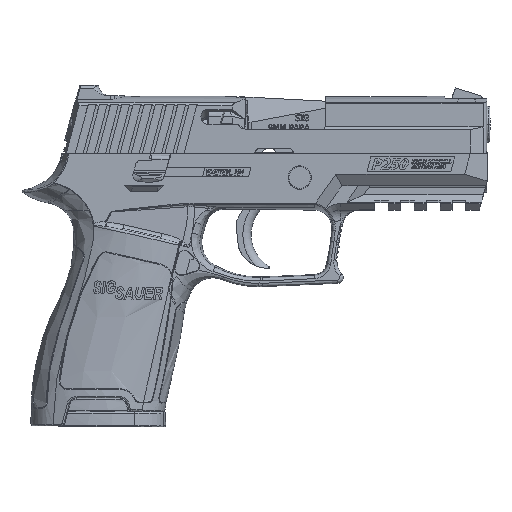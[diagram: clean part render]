
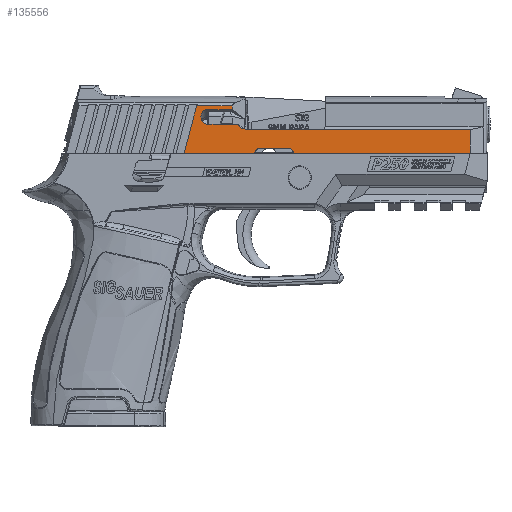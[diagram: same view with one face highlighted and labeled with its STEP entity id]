
A CAD part, top view. The second image highlights one B-rep face of the part: STEP entity #135556.
In plain terms, the highlighted planar face has unit normal (0, 0, 1).
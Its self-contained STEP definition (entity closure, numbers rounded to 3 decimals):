
#2922 = EDGE_CURVE ( 'NONE', #13814, #132730, #89528, .T. ) ;
#5060 = CARTESIAN_POINT ( 'NONE',  ( 76.306, -5.512, 13.392 ) ) ;
#7106 = CARTESIAN_POINT ( 'NONE',  ( -25.864, 5.823, 13.392 ) ) ;
#8354 = LINE ( 'NONE', #92009, #197966 ) ;
#10032 = VECTOR ( 'NONE', #90291, 1000. ) ;
#10388 = DIRECTION ( 'NONE',  ( -1., 0., 0. ) ) ;
#10726 = CIRCLE ( 'NONE', #40837, 1.892 ) ;
#12223 = VECTOR ( 'NONE', #10388, 1000. ) ;
#13460 = DIRECTION ( 'NONE',  ( 1., 0., 0. ) ) ;
#13528 = DIRECTION ( 'NONE',  ( 0., 0., -1. ) ) ;
#13814 = VERTEX_POINT ( 'NONE', #211452 ) ;
#14799 = CARTESIAN_POINT ( 'NONE',  ( 76.306, -1.88, 13.392 ) ) ;
#18044 = LINE ( 'NONE', #211913, #12223 ) ;
#18576 = VECTOR ( 'NONE', #13460, 1000. ) ;
#20163 = CARTESIAN_POINT ( 'NONE',  ( -16.059, 7.282, 13.392 ) ) ;
#24333 = LINE ( 'NONE', #105023, #18576 ) ;
#29088 = VECTOR ( 'NONE', #121950, 1000. ) ;
#29481 = VERTEX_POINT ( 'NONE', #107072 ) ;
#31237 = DIRECTION ( 'NONE',  ( 0., 1., 0. ) ) ;
#31293 = DIRECTION ( 'NONE',  ( 0., 0., -1. ) ) ;
#32846 = VERTEX_POINT ( 'NONE', #14799 ) ;
#38443 = CARTESIAN_POINT ( 'NONE',  ( -11.049, -1.88, 13.392 ) ) ;
#40493 = EDGE_CURVE ( 'NONE', #134322, #143446, #10726, .T. ) ;
#40837 = AXIS2_PLACEMENT_3D ( 'NONE', #123600, #13528, #142074 ) ;
#45986 = LINE ( 'NONE', #68827, #132365 ) ;
#46815 = AXIS2_PLACEMENT_3D ( 'NONE', #141336, #31293, #159759 ) ;
#49719 = CARTESIAN_POINT ( 'NONE',  ( -11.049, 1.499, 13.392 ) ) ;
#50342 = EDGE_CURVE ( 'NONE', #98184, #13814, #45986, .T. ) ;
#51182 = CARTESIAN_POINT ( 'NONE',  ( -33.313, -5.74, 13.392 ) ) ;
#51683 = CARTESIAN_POINT ( 'NONE',  ( 18.479, -1.88, 13.392 ) ) ;
#51698 = ORIENTED_EDGE ( 'NONE', *, *, #138721, .T. ) ;
#51825 = EDGE_CURVE ( 'NONE', #29481, #180648, #100212, .T. ) ;
#55468 = ORIENTED_EDGE ( 'NONE', *, *, #212171, .T. ) ;
#60237 = ORIENTED_EDGE ( 'NONE', *, *, #66510, .T. ) ;
#60846 = EDGE_CURVE ( 'NONE', #177034, #98184, #181710, .T. ) ;
#61339 = EDGE_CURVE ( 'NONE', #132730, #151941, #153221, .T. ) ;
#61347 = DIRECTION ( 'NONE',  ( 1., 0., 0. ) ) ;
#64230 = CARTESIAN_POINT ( 'NONE',  ( -30.436, 0.241, 13.392 ) ) ;
#66371 = LINE ( 'NONE', #51182, #29088 ) ;
#66510 = EDGE_CURVE ( 'NONE', #108976, #29481, #200389, .T. ) ;
#68212 = DIRECTION ( 'NONE',  ( -0.574, -0.819, 0. ) ) ;
#68827 = CARTESIAN_POINT ( 'NONE',  ( -11.049, 5.512, 13.392 ) ) ;
#71782 = CARTESIAN_POINT ( 'NONE',  ( 0., 5.823, 13.392 ) ) ;
#73894 = VERTEX_POINT ( 'NONE', #20163 ) ;
#76267 = ORIENTED_EDGE ( 'NONE', *, *, #149920, .T. ) ;
#78929 = CARTESIAN_POINT ( 'NONE',  ( -5.524, -1.88, 13.392 ) ) ;
#79886 = ORIENTED_EDGE ( 'NONE', *, *, #177039, .T. ) ;
#82765 = CARTESIAN_POINT ( 'NONE',  ( -30.436, 5.823, 13.392 ) ) ;
#84034 = VECTOR ( 'NONE', #188940, 1000. ) ;
#86768 = VERTEX_POINT ( 'NONE', #7106 ) ;
#87944 = EDGE_CURVE ( 'NONE', #211106, #134322, #24333, .T. ) ;
#89528 = CIRCLE ( 'NONE', #101850, 3.175 ) ;
#90291 = DIRECTION ( 'NONE',  ( 1., 0., 0. ) ) ;
#92009 = CARTESIAN_POINT ( 'NONE',  ( -10.287, 7.282, 13.392 ) ) ;
#92704 = EDGE_CURVE ( 'NONE', #143446, #108976, #215526, .T. ) ;
#93083 = CARTESIAN_POINT ( 'NONE',  ( -25.864, 0.241, 13.392 ) ) ;
#94252 = EDGE_CURVE ( 'NONE', #129541, #73894, #134827, .T. ) ;
#98107 = CARTESIAN_POINT ( 'NONE',  ( -29.824, 7.282, 13.392 ) ) ;
#98184 = VERTEX_POINT ( 'NONE', #38443 ) ;
#100212 = LINE ( 'NONE', #238475, #105996 ) ;
#101850 = AXIS2_PLACEMENT_3D ( 'NONE', #49719, #178216, #68212 ) ;
#104007 = EDGE_CURVE ( 'NONE', #32846, #177034, #18044, .T. ) ;
#105023 = CARTESIAN_POINT ( 'NONE',  ( 82.626, -11.024, 13.392 ) ) ;
#105996 = VECTOR ( 'NONE', #165419, 1000. ) ;
#106846 = VECTOR ( 'NONE', #172543, 1000. ) ;
#107072 = CARTESIAN_POINT ( 'NONE',  ( 7.696, -11.024, 13.392 ) ) ;
#108976 = VERTEX_POINT ( 'NONE', #150708 ) ;
#115071 = DIRECTION ( 'NONE',  ( 0., 1., 0. ) ) ;
#121950 = DIRECTION ( 'NONE',  ( -0.259, -0.966, 0. ) ) ;
#123600 = CARTESIAN_POINT ( 'NONE',  ( -5.347, -11.024, 13.392 ) ) ;
#126146 = ORIENTED_EDGE ( 'NONE', *, *, #94252, .T. ) ;
#126937 = EDGE_CURVE ( 'NONE', #180648, #32846, #166859, .T. ) ;
#127649 = DIRECTION ( 'NONE',  ( 1., 0., 0. ) ) ;
#129541 = VERTEX_POINT ( 'NONE', #170852 ) ;
#132365 = VECTOR ( 'NONE', #161971, 1000. ) ;
#132730 = VERTEX_POINT ( 'NONE', #227591 ) ;
#134322 = VERTEX_POINT ( 'NONE', #145056 ) ;
#134827 = LINE ( 'NONE', #141280, #183573 ) ;
#135556 = ADVANCED_FACE ( 'NONE', ( #208088 ), #219091, .T. ) ;
#138721 = EDGE_CURVE ( 'NONE', #147623, #211106, #66371, .T. ) ;
#139306 = CARTESIAN_POINT ( 'NONE',  ( -34.729, -11.024, 13.392 ) ) ;
#141280 = CARTESIAN_POINT ( 'NONE',  ( -16.059, 4.602, 13.392 ) ) ;
#141336 = CARTESIAN_POINT ( 'NONE',  ( 5.804, -11.024, 13.392 ) ) ;
#142074 = DIRECTION ( 'NONE',  ( 0., 1., 0. ) ) ;
#142079 = EDGE_LOOP ( 'NONE', ( #76267, #51698, #184163, #158860, #164573, #60237, #157191, #203242, #181123, #195046, #209443, #165718, #181007, #55468, #79886, #126146 ) ) ;
#143446 = VERTEX_POINT ( 'NONE', #213743 ) ;
#145056 = CARTESIAN_POINT ( 'NONE',  ( -7.239, -11.024, 13.392 ) ) ;
#147623 = VERTEX_POINT ( 'NONE', #98107 ) ;
#149920 = EDGE_CURVE ( 'NONE', #73894, #147623, #8354, .T. ) ;
#150708 = CARTESIAN_POINT ( 'NONE',  ( 5.804, -9.131, 13.392 ) ) ;
#151941 = VERTEX_POINT ( 'NONE', #93083 ) ;
#153221 = LINE ( 'NONE', #190978, #106846 ) ;
#156608 = LINE ( 'NONE', #71782, #10032 ) ;
#157191 = ORIENTED_EDGE ( 'NONE', *, *, #51825, .T. ) ;
#158860 = ORIENTED_EDGE ( 'NONE', *, *, #40493, .T. ) ;
#159759 = DIRECTION ( 'NONE',  ( 1., 0., 0. ) ) ;
#160980 = VECTOR ( 'NONE', #61347, 1000. ) ;
#161971 = DIRECTION ( 'NONE',  ( 0., 1., 0. ) ) ;
#163719 = CARTESIAN_POINT ( 'NONE',  ( 0., 0., 13.392 ) ) ;
#164573 = ORIENTED_EDGE ( 'NONE', *, *, #92704, .T. ) ;
#165419 = DIRECTION ( 'NONE',  ( 1., 0., 0. ) ) ;
#165718 = ORIENTED_EDGE ( 'NONE', *, *, #2922, .T. ) ;
#165897 = DIRECTION ( 'NONE',  ( -1., 0., 0. ) ) ;
#166859 = LINE ( 'NONE', #5060, #172572 ) ;
#170852 = CARTESIAN_POINT ( 'NONE',  ( -16.059, 5.823, 13.392 ) ) ;
#172543 = DIRECTION ( 'NONE',  ( -1., 0., 0. ) ) ;
#172572 = VECTOR ( 'NONE', #115071, 1000. ) ;
#174250 = CARTESIAN_POINT ( 'NONE',  ( -25.864, 0.241, 13.392 ) ) ;
#177034 = VERTEX_POINT ( 'NONE', #51683 ) ;
#177039 = EDGE_CURVE ( 'NONE', #86768, #129541, #156608, .T. ) ;
#178216 = DIRECTION ( 'NONE',  ( 0., 0., -1. ) ) ;
#180648 = VERTEX_POINT ( 'NONE', #224640 ) ;
#181007 = ORIENTED_EDGE ( 'NONE', *, *, #61339, .T. ) ;
#181123 = ORIENTED_EDGE ( 'NONE', *, *, #104007, .T. ) ;
#181710 = LINE ( 'NONE', #78929, #84034 ) ;
#183573 = VECTOR ( 'NONE', #31237, 1000. ) ;
#184163 = ORIENTED_EDGE ( 'NONE', *, *, #87944, .T. ) ;
#188940 = DIRECTION ( 'NONE',  ( -1., 0., 0. ) ) ;
#190978 = CARTESIAN_POINT ( 'NONE',  ( 0., 0.241, 13.392 ) ) ;
#195046 = ORIENTED_EDGE ( 'NONE', *, *, #60846, .T. ) ;
#197966 = VECTOR ( 'NONE', #165897, 1000. ) ;
#200389 = CIRCLE ( 'NONE', #46815, 1.892 ) ;
#203242 = ORIENTED_EDGE ( 'NONE', *, *, #126937, .T. ) ;
#206339 =( BOUNDED_CURVE ( )  B_SPLINE_CURVE ( 3, ( #174250, #64230, #82765, #211164 ),
 .UNSPECIFIED., .F., .T. ) 
 B_SPLINE_CURVE_WITH_KNOTS ( ( 4, 4 ),
 ( 3.142, 6.283 ),
 .UNSPECIFIED. ) 
 CURVE ( )  GEOMETRIC_REPRESENTATION_ITEM ( )  RATIONAL_B_SPLINE_CURVE ( ( 1., 0.333, 0.333, 1. ) ) 
 REPRESENTATION_ITEM ( '' )  );
#208088 = FACE_OUTER_BOUND ( 'NONE', #142079, .T. ) ;
#209113 = CARTESIAN_POINT ( 'NONE',  ( -2.673, -9.131, 13.392 ) ) ;
#209443 = ORIENTED_EDGE ( 'NONE', *, *, #50342, .T. ) ;
#211106 = VERTEX_POINT ( 'NONE', #139306 ) ;
#211164 = CARTESIAN_POINT ( 'NONE',  ( -25.864, 5.823, 13.392 ) ) ;
#211452 = CARTESIAN_POINT ( 'NONE',  ( -11.049, -1.676, 13.392 ) ) ;
#211913 = CARTESIAN_POINT ( 'NONE',  ( -5.524, -1.88, 13.392 ) ) ;
#212171 = EDGE_CURVE ( 'NONE', #151941, #86768, #206339, .T. ) ;
#213743 = CARTESIAN_POINT ( 'NONE',  ( -5.347, -9.131, 13.392 ) ) ;
#215526 = LINE ( 'NONE', #209113, #160980 ) ;
#219091 = PLANE ( 'NONE',  #236616 ) ;
#224640 = CARTESIAN_POINT ( 'NONE',  ( 76.306, -11.024, 13.392 ) ) ;
#227591 = CARTESIAN_POINT ( 'NONE',  ( -13.964, 0.241, 13.392 ) ) ;
#236616 = AXIS2_PLACEMENT_3D ( 'NONE', #163719, #237614, #127649 ) ;
#237614 = DIRECTION ( 'NONE',  ( 0., 0., 1. ) ) ;
#238475 = CARTESIAN_POINT ( 'NONE',  ( 82.626, -11.024, 13.392 ) ) ;
